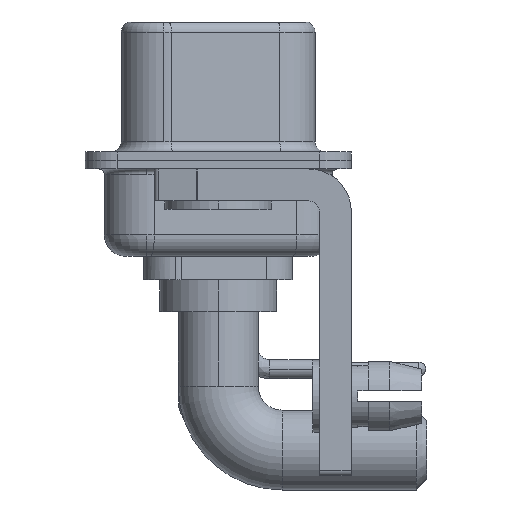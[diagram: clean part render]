
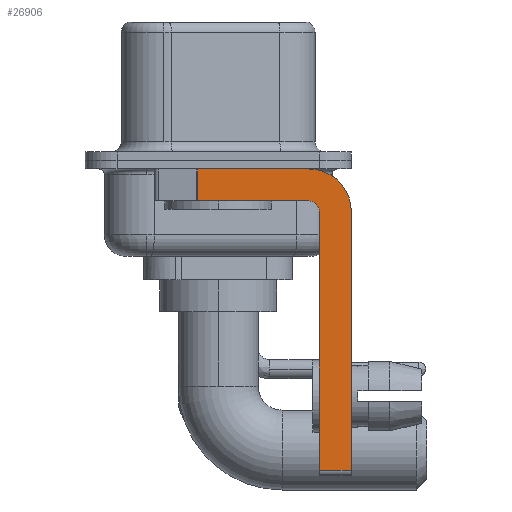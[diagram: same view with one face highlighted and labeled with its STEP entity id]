
A CAD part, left-side view. The second image highlights one B-rep face of the part: STEP entity #26906.
In plain terms, the highlighted planar face has unit normal (-1, 0, 0).
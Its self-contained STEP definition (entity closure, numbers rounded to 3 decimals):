
#182 = DIRECTION ( 'NONE',  ( -1., 0., 0. ) ) ;
#1102 = VECTOR ( 'NONE', #4851, 1000. ) ;
#1357 = VERTEX_POINT ( 'NONE', #16208 ) ;
#1395 = VECTOR ( 'NONE', #12534, 1000. ) ;
#1649 = LINE ( 'NONE', #9771, #10567 ) ;
#1979 = AXIS2_PLACEMENT_3D ( 'NONE', #4545, #4677, #2615 ) ;
#2591 = DIRECTION ( 'NONE',  ( 0., 0., -1. ) ) ;
#2615 = DIRECTION ( 'NONE',  ( 0., 0., -1. ) ) ;
#3062 = CARTESIAN_POINT ( 'NONE',  ( -2.9, -6.25, -2.4 ) ) ;
#4469 = EDGE_CURVE ( 'NONE', #21854, #15309, #25839, .T. ) ;
#4545 = CARTESIAN_POINT ( 'NONE',  ( -2.9, -4.25, -2.4 ) ) ;
#4677 = DIRECTION ( 'NONE',  ( 1., 0., 0. ) ) ;
#4851 = DIRECTION ( 'NONE',  ( 0., 0., -1. ) ) ;
#5222 = VERTEX_POINT ( 'NONE', #8502 ) ;
#5362 = LINE ( 'NONE', #15807, #15684 ) ;
#5605 = CARTESIAN_POINT ( 'NONE',  ( -2.9, -4.25, -2.4 ) ) ;
#6042 = DIRECTION ( 'NONE',  ( 0., -1., 0. ) ) ;
#6335 = ORIENTED_EDGE ( 'NONE', *, *, #18824, .F. ) ;
#6920 = AXIS2_PLACEMENT_3D ( 'NONE', #9728, #10504, #7648 ) ;
#7111 = LINE ( 'NONE', #21400, #20351 ) ;
#7648 = DIRECTION ( 'NONE',  ( 0., 0., -1. ) ) ;
#7776 = LINE ( 'NONE', #21550, #9913 ) ;
#8502 = CARTESIAN_POINT ( 'NONE',  ( -2.9, -4.25, -0.4 ) ) ;
#8786 = ORIENTED_EDGE ( 'NONE', *, *, #26966, .F. ) ;
#9063 = AXIS2_PLACEMENT_3D ( 'NONE', #5605, #182, #13988 ) ;
#9612 = ORIENTED_EDGE ( 'NONE', *, *, #13300, .F. ) ;
#9677 = ORIENTED_EDGE ( 'NONE', *, *, #26209, .F. ) ;
#9728 = CARTESIAN_POINT ( 'NONE',  ( -2.9, -4.25, -2.4 ) ) ;
#9771 = CARTESIAN_POINT ( 'NONE',  ( -2.9, -4.25, -14.55 ) ) ;
#9913 = VECTOR ( 'NONE', #11930, 1000. ) ;
#10504 = DIRECTION ( 'NONE',  ( 1., 0., 0. ) ) ;
#10567 = VECTOR ( 'NONE', #6042, 1000. ) ;
#11930 = DIRECTION ( 'NONE',  ( 0., -1., 0. ) ) ;
#11964 = VERTEX_POINT ( 'NONE', #3062 ) ;
#12507 = EDGE_CURVE ( 'NONE', #15003, #17783, #1649, .T. ) ;
#12534 = DIRECTION ( 'NONE',  ( 0., 0., 1. ) ) ;
#12638 = CIRCLE ( 'NONE', #9063, 0.5 ) ;
#12692 = PLANE ( 'NONE',  #6920 ) ;
#12979 = ORIENTED_EDGE ( 'NONE', *, *, #17497, .F. ) ;
#13300 = EDGE_CURVE ( 'NONE', #15003, #1357, #14593, .T. ) ;
#13668 = CARTESIAN_POINT ( 'NONE',  ( -2.9, 0.978, -1.9 ) ) ;
#13852 = FACE_OUTER_BOUND ( 'NONE', #20075, .T. ) ;
#13988 = DIRECTION ( 'NONE',  ( 0., 0., 1. ) ) ;
#14593 = LINE ( 'NONE', #24462, #1395 ) ;
#15003 = VERTEX_POINT ( 'NONE', #27098 ) ;
#15146 = CIRCLE ( 'NONE', #1979, 2. ) ;
#15309 = VERTEX_POINT ( 'NONE', #13668 ) ;
#15552 = ORIENTED_EDGE ( 'NONE', *, *, #21519, .F. ) ;
#15684 = VECTOR ( 'NONE', #21835, 1000. ) ;
#15807 = CARTESIAN_POINT ( 'NONE',  ( -2.9, -4.25, -1.9 ) ) ;
#16208 = CARTESIAN_POINT ( 'NONE',  ( -2.9, -4.75, -2.4 ) ) ;
#16441 = CARTESIAN_POINT ( 'NONE',  ( -2.9, -4.25, -1.9 ) ) ;
#17497 = EDGE_CURVE ( 'NONE', #21854, #5222, #7776, .T. ) ;
#17675 = VERTEX_POINT ( 'NONE', #16441 ) ;
#17783 = VERTEX_POINT ( 'NONE', #21619 ) ;
#18511 = CARTESIAN_POINT ( 'NONE',  ( -2.9, 0.978, -0.4 ) ) ;
#18824 = EDGE_CURVE ( 'NONE', #5222, #11964, #15146, .T. ) ;
#19547 = CARTESIAN_POINT ( 'NONE',  ( -2.9, 0.978, -1.9 ) ) ;
#20075 = EDGE_LOOP ( 'NONE', ( #12979, #24391, #9677, #8786, #9612, #20999, #15552, #6335 ) ) ;
#20351 = VECTOR ( 'NONE', #2591, 1000. ) ;
#20999 = ORIENTED_EDGE ( 'NONE', *, *, #12507, .T. ) ;
#21400 = CARTESIAN_POINT ( 'NONE',  ( -2.9, -6.25, -2.4 ) ) ;
#21519 = EDGE_CURVE ( 'NONE', #11964, #17783, #7111, .T. ) ;
#21550 = CARTESIAN_POINT ( 'NONE',  ( -2.9, 3., -0.4 ) ) ;
#21619 = CARTESIAN_POINT ( 'NONE',  ( -2.9, -6.25, -14.55 ) ) ;
#21835 = DIRECTION ( 'NONE',  ( 0., 1., 0. ) ) ;
#21854 = VERTEX_POINT ( 'NONE', #18511 ) ;
#24391 = ORIENTED_EDGE ( 'NONE', *, *, #4469, .T. ) ;
#24462 = CARTESIAN_POINT ( 'NONE',  ( -2.9, -4.75, -14.8 ) ) ;
#25839 = LINE ( 'NONE', #19547, #1102 ) ;
#26209 = EDGE_CURVE ( 'NONE', #17675, #15309, #5362, .T. ) ;
#26906 = ADVANCED_FACE ( 'NONE', ( #13852 ), #12692, .F. ) ;
#26966 = EDGE_CURVE ( 'NONE', #1357, #17675, #12638, .T. ) ;
#27098 = CARTESIAN_POINT ( 'NONE',  ( -2.9, -4.75, -14.55 ) ) ;
